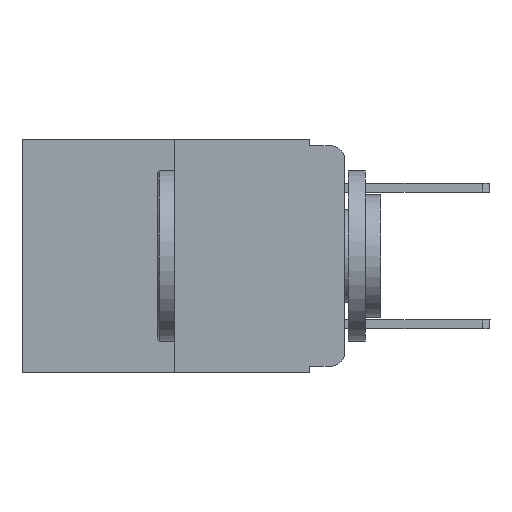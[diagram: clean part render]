
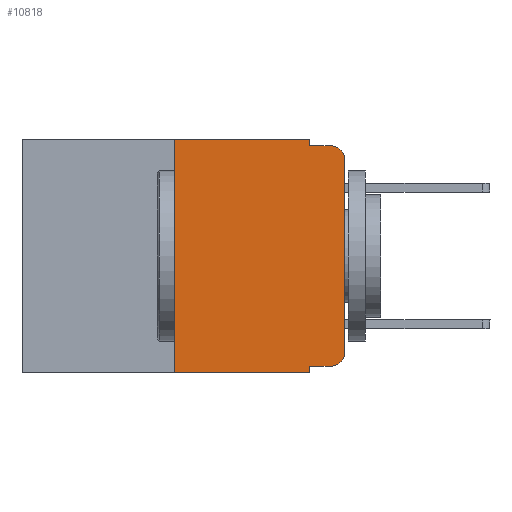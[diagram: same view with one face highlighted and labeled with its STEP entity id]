
A CAD part, left-side view. The second image highlights one B-rep face of the part: STEP entity #10818.
In plain terms, the highlighted planar face has unit normal (-1, 0, 0).
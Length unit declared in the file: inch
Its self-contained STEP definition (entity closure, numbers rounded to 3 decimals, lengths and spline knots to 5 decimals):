
#318 = VERTEX_POINT ( 'NONE', #11909 ) ;
#939 = DIRECTION ( 'NONE',  ( 0., -1., 0. ) ) ;
#1464 = CARTESIAN_POINT ( 'NONE',  ( 0., 0.051, -0.333 ) ) ;
#1499 = DIRECTION ( 'NONE',  ( 0., -1., 0. ) ) ;
#2110 = FACE_OUTER_BOUND ( 'NONE', #13996, .T. ) ;
#2243 = CARTESIAN_POINT ( 'NONE',  ( 0., 0.25, 0. ) ) ;
#2269 = VECTOR ( 'NONE', #12664, 39.37008 ) ;
#2325 = CARTESIAN_POINT ( 'NONE',  ( 0., 0.25, -0.343 ) ) ;
#2367 = CARTESIAN_POINT ( 'NONE',  ( 0., 0.02, -0.01 ) ) ;
#3019 = CARTESIAN_POINT ( 'NONE',  ( 0., 0.051, -0.01 ) ) ;
#3046 = AXIS2_PLACEMENT_3D ( 'NONE', #14610, #3430, #6844 ) ;
#3049 = VECTOR ( 'NONE', #1499, 39.37008 ) ;
#3197 = DIRECTION ( 'NONE',  ( -1., 0., 0. ) ) ;
#3234 = DIRECTION ( 'NONE',  ( 0., 0., -1. ) ) ;
#3430 = DIRECTION ( 'NONE',  ( -1., 0., 0. ) ) ;
#3545 = DIRECTION ( 'NONE',  ( 0., -1., 0. ) ) ;
#3596 = ORIENTED_EDGE ( 'NONE', *, *, #12076, .T. ) ;
#3846 = VERTEX_POINT ( 'NONE', #13672 ) ;
#3885 = CARTESIAN_POINT ( 'NONE',  ( 0., 0.051, 0. ) ) ;
#4029 = AXIS2_PLACEMENT_3D ( 'NONE', #14492, #13367, #3234 ) ;
#4657 = LINE ( 'NONE', #5703, #9110 ) ;
#4726 = ORIENTED_EDGE ( 'NONE', *, *, #6048, .T. ) ;
#4991 = VERTEX_POINT ( 'NONE', #3019 ) ;
#5073 = EDGE_CURVE ( 'NONE', #4991, #8649, #10292, .T. ) ;
#5114 = AXIS2_PLACEMENT_3D ( 'NONE', #13625, #3197, #9039 ) ;
#5406 = CARTESIAN_POINT ( 'NONE',  ( 0., 0.473, -0.343 ) ) ;
#5418 = ORIENTED_EDGE ( 'NONE', *, *, #12057, .T. ) ;
#5466 = PLANE ( 'NONE',  #4029 ) ;
#5561 = LINE ( 'NONE', #5630, #10716 ) ;
#5601 = VERTEX_POINT ( 'NONE', #2325 ) ;
#5630 = CARTESIAN_POINT ( 'NONE',  ( 0., 0.051, 0. ) ) ;
#5703 = CARTESIAN_POINT ( 'NONE',  ( 0., 0.473, 0. ) ) ;
#5737 = ORIENTED_EDGE ( 'NONE', *, *, #14208, .F. ) ;
#5971 = ORIENTED_EDGE ( 'NONE', *, *, #10103, .T. ) ;
#5990 = ORIENTED_EDGE ( 'NONE', *, *, #8000, .F. ) ;
#6041 = DIRECTION ( 'NONE',  ( 0., 0., -1. ) ) ;
#6048 = EDGE_CURVE ( 'NONE', #6586, #3846, #10643, .T. ) ;
#6298 = CIRCLE ( 'NONE', #5114, 0.02 ) ;
#6586 = VERTEX_POINT ( 'NONE', #7916 ) ;
#6600 = EDGE_CURVE ( 'NONE', #11163, #12351, #4657, .T. ) ;
#6601 = CARTESIAN_POINT ( 'NONE',  ( 0., 0.051, -0.333 ) ) ;
#6844 = DIRECTION ( 'NONE',  ( 0., 0., -1. ) ) ;
#7428 = VECTOR ( 'NONE', #6041, 39.37008 ) ;
#7636 = CARTESIAN_POINT ( 'NONE',  ( 0., 0., 0. ) ) ;
#7694 = ORIENTED_EDGE ( 'NONE', *, *, #13174, .F. ) ;
#7878 = EDGE_CURVE ( 'NONE', #318, #8649, #6298, .T. ) ;
#7916 = CARTESIAN_POINT ( 'NONE',  ( 0., 0.02, -0.333 ) ) ;
#8000 = EDGE_CURVE ( 'NONE', #5601, #11163, #8305, .T. ) ;
#8305 = LINE ( 'NONE', #10459, #2269 ) ;
#8649 = VERTEX_POINT ( 'NONE', #2367 ) ;
#8730 = CARTESIAN_POINT ( 'NONE',  ( 0., 0.051, -0.343 ) ) ;
#8807 = LINE ( 'NONE', #7636, #13032 ) ;
#9039 = DIRECTION ( 'NONE',  ( 0., 0., -1. ) ) ;
#9110 = VECTOR ( 'NONE', #3545, 39.37008 ) ;
#9164 = DIRECTION ( 'NONE',  ( 0., -1., 0. ) ) ;
#9429 = LINE ( 'NONE', #3885, #7428 ) ;
#10103 = EDGE_CURVE ( 'NONE', #5601, #11988, #11922, .T. ) ;
#10292 = LINE ( 'NONE', #14578, #10380 ) ;
#10380 = VECTOR ( 'NONE', #9164, 39.37008 ) ;
#10434 = VERTEX_POINT ( 'NONE', #1464 ) ;
#10459 = CARTESIAN_POINT ( 'NONE',  ( 0., 0.25, 0. ) ) ;
#10494 = ORIENTED_EDGE ( 'NONE', *, *, #5073, .F. ) ;
#10643 = CIRCLE ( 'NONE', #3046, 0.02 ) ;
#10716 = VECTOR ( 'NONE', #12433, 39.37008 ) ;
#10818 = ADVANCED_FACE ( 'NONE', ( #2110 ), #5466, .F. ) ;
#11163 = VERTEX_POINT ( 'NONE', #2243 ) ;
#11536 = ORIENTED_EDGE ( 'NONE', *, *, #6600, .F. ) ;
#11638 = VECTOR ( 'NONE', #939, 39.37008 ) ;
#11909 = CARTESIAN_POINT ( 'NONE',  ( 0., 0., -0.03 ) ) ;
#11922 = LINE ( 'NONE', #5406, #3049 ) ;
#11988 = VERTEX_POINT ( 'NONE', #8730 ) ;
#11995 = LINE ( 'NONE', #6601, #11638 ) ;
#12057 = EDGE_CURVE ( 'NONE', #10434, #6586, #11995, .T. ) ;
#12076 = EDGE_CURVE ( 'NONE', #3846, #318, #8807, .T. ) ;
#12351 = VERTEX_POINT ( 'NONE', #13366 ) ;
#12433 = DIRECTION ( 'NONE',  ( 0., 0., -1. ) ) ;
#12664 = DIRECTION ( 'NONE',  ( 0., 0., 1. ) ) ;
#13032 = VECTOR ( 'NONE', #13317, 39.37008 ) ;
#13174 = EDGE_CURVE ( 'NONE', #12351, #4991, #5561, .T. ) ;
#13317 = DIRECTION ( 'NONE',  ( 0., 0., 1. ) ) ;
#13366 = CARTESIAN_POINT ( 'NONE',  ( 0., 0.051, 0. ) ) ;
#13367 = DIRECTION ( 'NONE',  ( 1., 0., 0. ) ) ;
#13456 = ORIENTED_EDGE ( 'NONE', *, *, #7878, .T. ) ;
#13625 = CARTESIAN_POINT ( 'NONE',  ( 0., 0.02, -0.03 ) ) ;
#13672 = CARTESIAN_POINT ( 'NONE',  ( 0., 0., -0.313 ) ) ;
#13996 = EDGE_LOOP ( 'NONE', ( #3596, #13456, #10494, #7694, #11536, #5990, #5971, #5737, #5418, #4726 ) ) ;
#14208 = EDGE_CURVE ( 'NONE', #10434, #11988, #9429, .T. ) ;
#14492 = CARTESIAN_POINT ( 'NONE',  ( 0., 0.473, 0. ) ) ;
#14578 = CARTESIAN_POINT ( 'NONE',  ( 0., 0.051, -0.01 ) ) ;
#14610 = CARTESIAN_POINT ( 'NONE',  ( 0., 0.02, -0.313 ) ) ;
